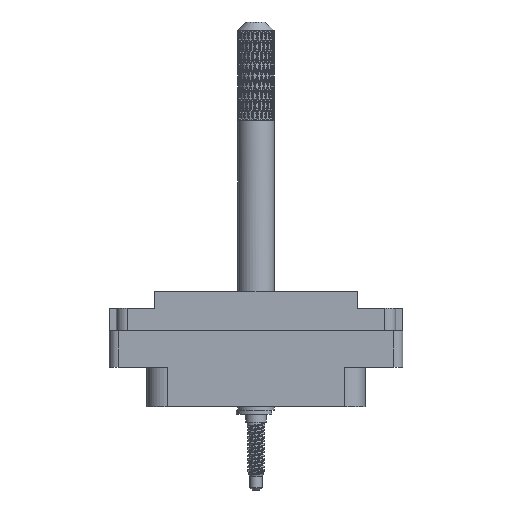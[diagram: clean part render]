
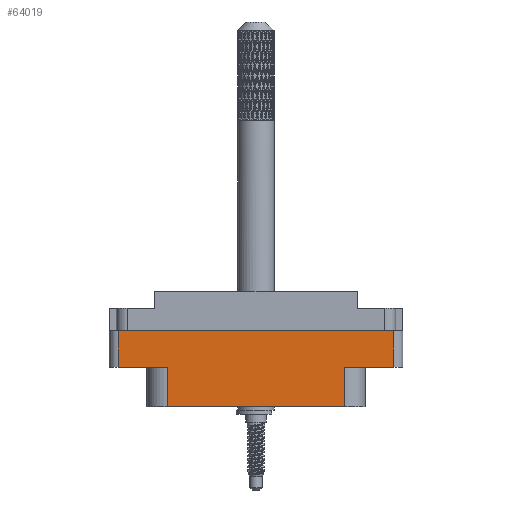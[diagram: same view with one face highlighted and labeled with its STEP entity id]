
A CAD part, front view. The second image highlights one B-rep face of the part: STEP entity #64019.
In plain terms, the highlighted planar face has unit normal (0, -1, 0).
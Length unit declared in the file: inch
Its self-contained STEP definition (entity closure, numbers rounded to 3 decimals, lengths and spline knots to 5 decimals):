
#245 = CARTESIAN_POINT ( 'NONE',  ( 0.938, -0.438, -0.268 ) ) ;
#680 = CARTESIAN_POINT ( 'NONE',  ( -0.604, -0.438, -0.789 ) ) ;
#1082 = CARTESIAN_POINT ( 'NONE',  ( 0., -0.438, -0.52 ) ) ;
#4551 = CARTESIAN_POINT ( 'NONE',  ( 0.938, -0.438, -0.789 ) ) ;
#5543 = EDGE_CURVE ( 'NONE', #8726, #59990, #82557, .T. ) ;
#6046 = CARTESIAN_POINT ( 'NONE',  ( -1., -0.438, -0.789 ) ) ;
#7404 = DIRECTION ( 'NONE',  ( 1., 0., 0. ) ) ;
#7987 = LINE ( 'NONE', #83530, #34355 ) ;
#8726 = VERTEX_POINT ( 'NONE', #21800 ) ;
#10724 = VERTEX_POINT ( 'NONE', #22398 ) ;
#11281 = LINE ( 'NONE', #13948, #26865 ) ;
#13948 = CARTESIAN_POINT ( 'NONE',  ( -0.938, -0.438, -0.789 ) ) ;
#14149 = VERTEX_POINT ( 'NONE', #53860 ) ;
#15186 = ORIENTED_EDGE ( 'NONE', *, *, #5543, .T. ) ;
#15342 = ORIENTED_EDGE ( 'NONE', *, *, #37380, .T. ) ;
#15374 = ORIENTED_EDGE ( 'NONE', *, *, #33138, .T. ) ;
#16524 = DIRECTION ( 'NONE',  ( 0., -1., 0. ) ) ;
#17547 = DIRECTION ( 'NONE',  ( -1., 0., 0. ) ) ;
#21800 = CARTESIAN_POINT ( 'NONE',  ( -0.604, -0.438, -0.52 ) ) ;
#22398 = CARTESIAN_POINT ( 'NONE',  ( 0.938, -0.438, -0.52 ) ) ;
#25348 = LINE ( 'NONE', #4551, #89129 ) ;
#26865 = VECTOR ( 'NONE', #44498, 39.37008 ) ;
#28429 = VECTOR ( 'NONE', #63629, 39.37008 ) ;
#30026 = DIRECTION ( 'NONE',  ( 1., 0., 0. ) ) ;
#32573 = VECTOR ( 'NONE', #7404, 39.37008 ) ;
#33138 = EDGE_CURVE ( 'NONE', #34162, #97625, #53818, .T. ) ;
#33865 = CARTESIAN_POINT ( 'NONE',  ( 0., -0.438, -0.268 ) ) ;
#34162 = VERTEX_POINT ( 'NONE', #80196 ) ;
#34355 = VECTOR ( 'NONE', #30026, 39.37008 ) ;
#35011 = FACE_OUTER_BOUND ( 'NONE', #72505, .T. ) ;
#37380 = EDGE_CURVE ( 'NONE', #59990, #34162, #68730, .T. ) ;
#39781 = ORIENTED_EDGE ( 'NONE', *, *, #75578, .F. ) ;
#40065 = ORIENTED_EDGE ( 'NONE', *, *, #92553, .T. ) ;
#40343 = LINE ( 'NONE', #33865, #76522 ) ;
#40910 = DIRECTION ( 'NONE',  ( 1., 0., 0. ) ) ;
#44498 = DIRECTION ( 'NONE',  ( 0., 0., -1. ) ) ;
#44998 = PLANE ( 'NONE',  #49450 ) ;
#49450 = AXIS2_PLACEMENT_3D ( 'NONE', #6046, #16524, #60165 ) ;
#51073 = CARTESIAN_POINT ( 'NONE',  ( 0.604, -0.438, -0.52 ) ) ;
#52240 = VECTOR ( 'NONE', #17547, 39.37008 ) ;
#53466 = CARTESIAN_POINT ( 'NONE',  ( -1., -0.438, -0.789 ) ) ;
#53818 = LINE ( 'NONE', #60327, #73075 ) ;
#53860 = CARTESIAN_POINT ( 'NONE',  ( -0.938, -0.438, -0.268 ) ) ;
#54671 = EDGE_CURVE ( 'NONE', #70202, #8726, #7987, .T. ) ;
#57642 = DIRECTION ( 'NONE',  ( 0., 0., 1. ) ) ;
#59990 = VERTEX_POINT ( 'NONE', #680 ) ;
#60165 = DIRECTION ( 'NONE',  ( 0., 0., -1. ) ) ;
#60327 = CARTESIAN_POINT ( 'NONE',  ( 0.604, -0.438, -0.52 ) ) ;
#63629 = DIRECTION ( 'NONE',  ( 0., 0., -1. ) ) ;
#64019 = ADVANCED_FACE ( 'NONE', ( #35011 ), #44998, .T. ) ;
#64554 = EDGE_CURVE ( 'NONE', #10724, #69077, #25348, .T. ) ;
#66853 = CARTESIAN_POINT ( 'NONE',  ( -0.938, -0.438, -0.52 ) ) ;
#68409 = DIRECTION ( 'NONE',  ( 0., 0., 1. ) ) ;
#68730 = LINE ( 'NONE', #53466, #32573 ) ;
#69077 = VERTEX_POINT ( 'NONE', #245 ) ;
#70202 = VERTEX_POINT ( 'NONE', #66853 ) ;
#72505 = EDGE_LOOP ( 'NONE', ( #39781, #40065, #89301, #15186, #15342, #15374, #75749, #73414 ) ) ;
#73075 = VECTOR ( 'NONE', #68409, 39.37008 ) ;
#73414 = ORIENTED_EDGE ( 'NONE', *, *, #64554, .T. ) ;
#75578 = EDGE_CURVE ( 'NONE', #14149, #69077, #40343, .T. ) ;
#75749 = ORIENTED_EDGE ( 'NONE', *, *, #77117, .F. ) ;
#76522 = VECTOR ( 'NONE', #40910, 39.37008 ) ;
#77117 = EDGE_CURVE ( 'NONE', #10724, #97625, #96691, .T. ) ;
#80196 = CARTESIAN_POINT ( 'NONE',  ( 0.604, -0.438, -0.789 ) ) ;
#82557 = LINE ( 'NONE', #85837, #28429 ) ;
#83530 = CARTESIAN_POINT ( 'NONE',  ( 0., -0.438, -0.52 ) ) ;
#85837 = CARTESIAN_POINT ( 'NONE',  ( -0.604, -0.438, -0.789 ) ) ;
#89129 = VECTOR ( 'NONE', #57642, 39.37008 ) ;
#89301 = ORIENTED_EDGE ( 'NONE', *, *, #54671, .T. ) ;
#92553 = EDGE_CURVE ( 'NONE', #14149, #70202, #11281, .T. ) ;
#96691 = LINE ( 'NONE', #1082, #52240 ) ;
#97625 = VERTEX_POINT ( 'NONE', #51073 ) ;
